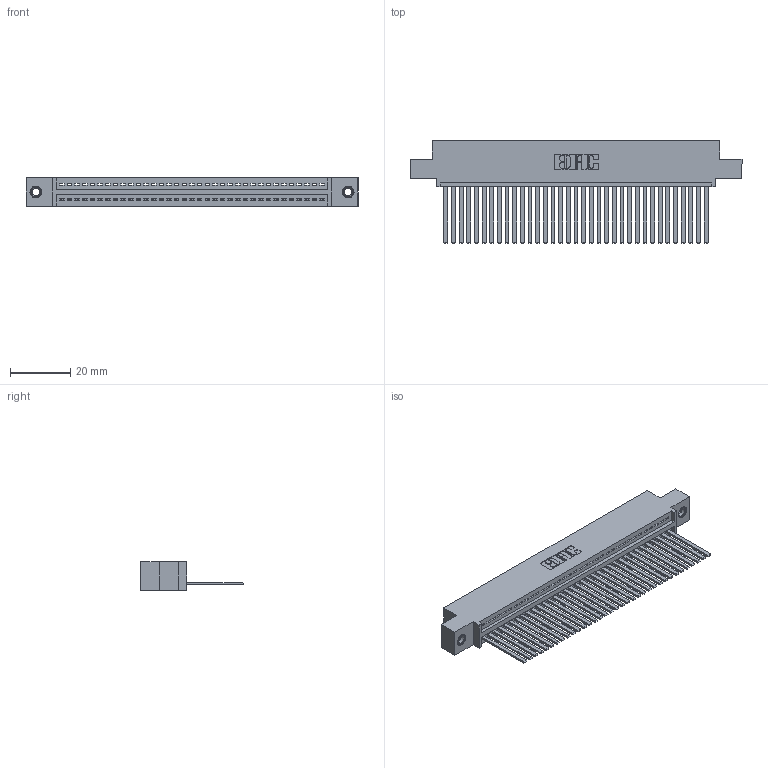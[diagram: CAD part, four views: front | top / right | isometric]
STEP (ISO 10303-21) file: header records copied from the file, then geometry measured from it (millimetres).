
FILE_DESCRIPTION (( 'STEP AP203' ), '1' );
FILE_NAME ('395-035-544-407.STEP', '2019-10-19T20:04:12', ( '' ), ( '' ), 'SwSTEP 2.0', 'SolidWorks 2016', '' );
FILE_SCHEMA (( 'CONFIG_CONTROL_DESIGN' ));
Length unit declared in the file: inch
Products named in the file (4): 345 Part_0.110 Offset - 0.156 Dia-TI; 345-292-001_345-293-144; 395-035-544-407; 345-250-001_345-250-005-103
Assembly tree (38 placements, depth 2):
  395-035-544-407
    345 Part_0.110 Offset - 0.156 Dia-TI
    345-292-001_345-293-144  x35
    345-250-001_345-250-005-103  x2
Bounding box: 110.11 x 33.96 x 9.4 mm (x, y, z)
Volume: 10719.4 mm3; surface area: 15481.3 mm2
Topology: 38 solids, 38 shells, 2010 faces, 6019 edges, 3958 vertices
Faces by surface type: plane 1376, cylinder 618, cone 12, torus 4
Entity records: 28418 total; most frequent: CARTESIAN_POINT 4904, ORIENTED_EDGE 4866, DIRECTION 4317, EDGE_CURVE 2433, VECTOR 2145, LINE 2145, VERTEX_POINT 1616, AXIS2_PLACEMENT_3D 1086
